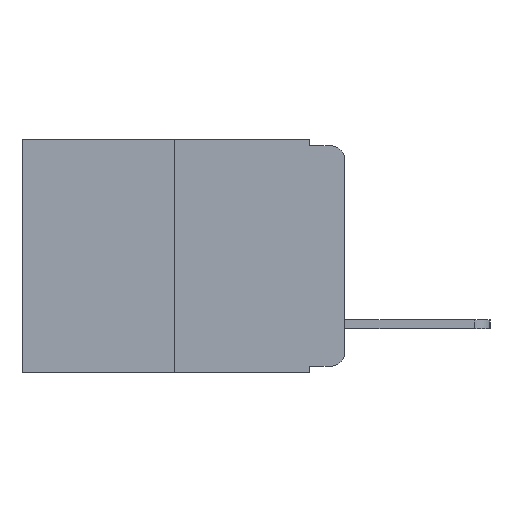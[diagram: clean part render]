
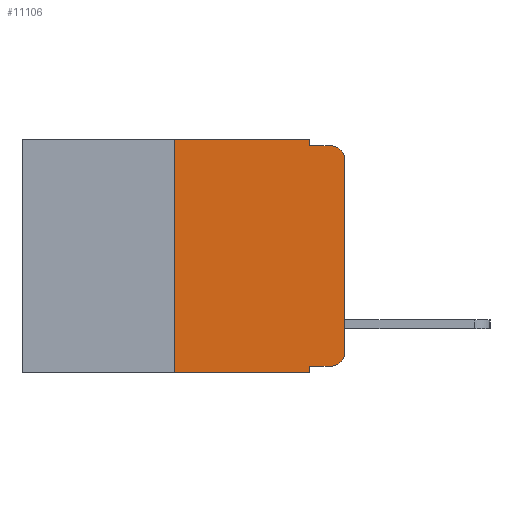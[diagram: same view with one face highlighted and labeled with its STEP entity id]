
A CAD part, left-side view. The second image highlights one B-rep face of the part: STEP entity #11106.
In plain terms, the highlighted planar face has unit normal (-1, 0, 0).
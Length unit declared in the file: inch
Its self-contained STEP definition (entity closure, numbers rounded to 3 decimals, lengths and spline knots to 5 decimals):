
#23 = VECTOR ( 'NONE', #1997, 39.37008 ) ;
#41 = LINE ( 'NONE', #2177, #10870 ) ;
#74 = CARTESIAN_POINT ( 'NONE',  ( 0., 0., -0.313 ) ) ;
#138 = VERTEX_POINT ( 'NONE', #4470 ) ;
#199 = VERTEX_POINT ( 'NONE', #8783 ) ;
#935 = ORIENTED_EDGE ( 'NONE', *, *, #12885, .T. ) ;
#968 = CARTESIAN_POINT ( 'NONE',  ( 0., 0.051, 0. ) ) ;
#1036 = EDGE_CURVE ( 'NONE', #6700, #4221, #2972, .T. ) ;
#1096 = DIRECTION ( 'NONE',  ( 0., 0., -1. ) ) ;
#1113 = CARTESIAN_POINT ( 'NONE',  ( 0., 0.25, 0. ) ) ;
#1255 = ORIENTED_EDGE ( 'NONE', *, *, #10306, .F. ) ;
#1504 = EDGE_CURVE ( 'NONE', #4419, #199, #8172, .T. ) ;
#1669 = CARTESIAN_POINT ( 'NONE',  ( 0., 0.02, -0.01 ) ) ;
#1930 = AXIS2_PLACEMENT_3D ( 'NONE', #8743, #2529, #9730 ) ;
#1997 = DIRECTION ( 'NONE',  ( 0., -1., 0. ) ) ;
#2034 = ORIENTED_EDGE ( 'NONE', *, *, #3650, .T. ) ;
#2177 = CARTESIAN_POINT ( 'NONE',  ( 0., 0.051, -0.333 ) ) ;
#2356 = ORIENTED_EDGE ( 'NONE', *, *, #9198, .F. ) ;
#2416 = ORIENTED_EDGE ( 'NONE', *, *, #1036, .T. ) ;
#2529 = DIRECTION ( 'NONE',  ( -1., 0., 0. ) ) ;
#2649 = VECTOR ( 'NONE', #13374, 39.37008 ) ;
#2805 = VERTEX_POINT ( 'NONE', #1669 ) ;
#2867 = DIRECTION ( 'NONE',  ( 0., -1., 0. ) ) ;
#2972 = LINE ( 'NONE', #7767, #2649 ) ;
#3096 = DIRECTION ( 'NONE',  ( 0., 0., 1. ) ) ;
#3132 = CARTESIAN_POINT ( 'NONE',  ( 0., 0.25, 0. ) ) ;
#3137 = VECTOR ( 'NONE', #10039, 39.37008 ) ;
#3354 = ORIENTED_EDGE ( 'NONE', *, *, #10720, .T. ) ;
#3388 = EDGE_CURVE ( 'NONE', #10461, #12256, #8670, .T. ) ;
#3505 = CARTESIAN_POINT ( 'NONE',  ( 0., 0.051, -0.343 ) ) ;
#3532 = ORIENTED_EDGE ( 'NONE', *, *, #1504, .T. ) ;
#3650 = EDGE_CURVE ( 'NONE', #138, #6586, #41, .T. ) ;
#3766 = CARTESIAN_POINT ( 'NONE',  ( 0., 0.051, 0. ) ) ;
#3854 = CIRCLE ( 'NONE', #1930, 0.02 ) ;
#4221 = VERTEX_POINT ( 'NONE', #3505 ) ;
#4248 = CARTESIAN_POINT ( 'NONE',  ( 0., 0.051, -0.01 ) ) ;
#4375 = DIRECTION ( 'NONE',  ( -1., 0., 0. ) ) ;
#4419 = VERTEX_POINT ( 'NONE', #74 ) ;
#4470 = CARTESIAN_POINT ( 'NONE',  ( 0., 0.051, -0.333 ) ) ;
#4602 = VERTEX_POINT ( 'NONE', #3132 ) ;
#4879 = VECTOR ( 'NONE', #9394, 39.37008 ) ;
#5157 = ORIENTED_EDGE ( 'NONE', *, *, #11955, .F. ) ;
#5394 = ORIENTED_EDGE ( 'NONE', *, *, #9015, .F. ) ;
#5445 = VECTOR ( 'NONE', #3096, 39.37008 ) ;
#5663 = CARTESIAN_POINT ( 'NONE',  ( 0., 0.02, -0.333 ) ) ;
#5834 = CARTESIAN_POINT ( 'NONE',  ( 0., 0.25, -0.343 ) ) ;
#6385 = LINE ( 'NONE', #10089, #11891 ) ;
#6586 = VERTEX_POINT ( 'NONE', #5663 ) ;
#6700 = VERTEX_POINT ( 'NONE', #5834 ) ;
#7252 = ORIENTED_EDGE ( 'NONE', *, *, #3388, .F. ) ;
#7335 = DIRECTION ( 'NONE',  ( 1., 0., 0. ) ) ;
#7767 = CARTESIAN_POINT ( 'NONE',  ( 0., 0.473, -0.343 ) ) ;
#8172 = LINE ( 'NONE', #13492, #5445 ) ;
#8670 = LINE ( 'NONE', #3766, #3137 ) ;
#8735 = AXIS2_PLACEMENT_3D ( 'NONE', #10523, #4375, #11582 ) ;
#8743 = CARTESIAN_POINT ( 'NONE',  ( 0., 0.02, -0.313 ) ) ;
#8783 = CARTESIAN_POINT ( 'NONE',  ( 0., 0., -0.03 ) ) ;
#8941 = CARTESIAN_POINT ( 'NONE',  ( 0., 0.051, -0.01 ) ) ;
#9015 = EDGE_CURVE ( 'NONE', #4602, #10461, #6385, .T. ) ;
#9198 = EDGE_CURVE ( 'NONE', #138, #4221, #9298, .T. ) ;
#9298 = LINE ( 'NONE', #968, #12043 ) ;
#9394 = DIRECTION ( 'NONE',  ( 0., 0., 1. ) ) ;
#9730 = DIRECTION ( 'NONE',  ( 0., 0., -1. ) ) ;
#9881 = CIRCLE ( 'NONE', #8735, 0.02 ) ;
#10004 = AXIS2_PLACEMENT_3D ( 'NONE', #12452, #7335, #1096 ) ;
#10039 = DIRECTION ( 'NONE',  ( 0., 0., -1. ) ) ;
#10089 = CARTESIAN_POINT ( 'NONE',  ( 0., 0.473, 0. ) ) ;
#10306 = EDGE_CURVE ( 'NONE', #12256, #2805, #10856, .T. ) ;
#10461 = VERTEX_POINT ( 'NONE', #12948 ) ;
#10523 = CARTESIAN_POINT ( 'NONE',  ( 0., 0.02, -0.03 ) ) ;
#10633 = LINE ( 'NONE', #1113, #4879 ) ;
#10720 = EDGE_CURVE ( 'NONE', #199, #2805, #9881, .T. ) ;
#10856 = LINE ( 'NONE', #4248, #23 ) ;
#10870 = VECTOR ( 'NONE', #12035, 39.37008 ) ;
#11106 = ADVANCED_FACE ( 'NONE', ( #12769 ), #11427, .F. ) ;
#11427 = PLANE ( 'NONE',  #10004 ) ;
#11474 = EDGE_LOOP ( 'NONE', ( #3532, #3354, #1255, #7252, #5394, #5157, #2416, #2356, #2034, #935 ) ) ;
#11582 = DIRECTION ( 'NONE',  ( 0., 0., -1. ) ) ;
#11891 = VECTOR ( 'NONE', #2867, 39.37008 ) ;
#11955 = EDGE_CURVE ( 'NONE', #6700, #4602, #10633, .T. ) ;
#12035 = DIRECTION ( 'NONE',  ( 0., -1., 0. ) ) ;
#12043 = VECTOR ( 'NONE', #12389, 39.37008 ) ;
#12256 = VERTEX_POINT ( 'NONE', #8941 ) ;
#12389 = DIRECTION ( 'NONE',  ( 0., 0., -1. ) ) ;
#12452 = CARTESIAN_POINT ( 'NONE',  ( 0., 0.473, 0. ) ) ;
#12769 = FACE_OUTER_BOUND ( 'NONE', #11474, .T. ) ;
#12885 = EDGE_CURVE ( 'NONE', #6586, #4419, #3854, .T. ) ;
#12948 = CARTESIAN_POINT ( 'NONE',  ( 0., 0.051, 0. ) ) ;
#13374 = DIRECTION ( 'NONE',  ( 0., -1., 0. ) ) ;
#13492 = CARTESIAN_POINT ( 'NONE',  ( 0., 0., 0. ) ) ;
